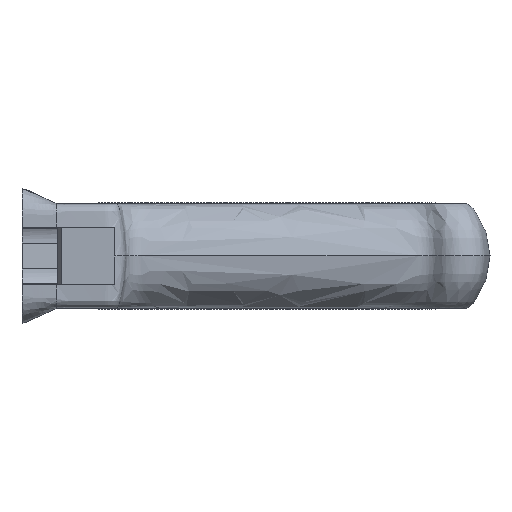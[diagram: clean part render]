
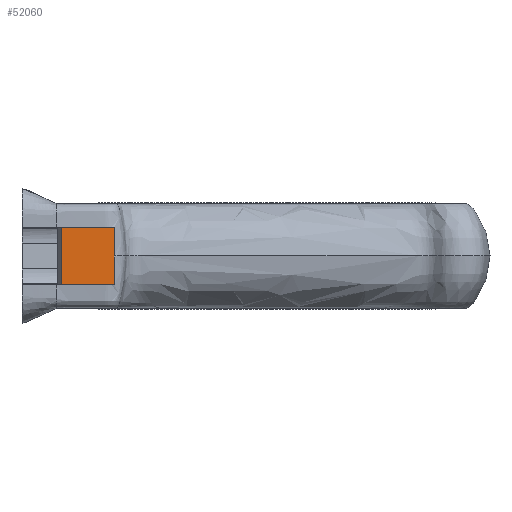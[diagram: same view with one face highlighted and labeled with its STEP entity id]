
A CAD part, left-side view. The second image highlights one B-rep face of the part: STEP entity #52060.
In plain terms, the highlighted planar face has unit normal (-1, 0, 0).
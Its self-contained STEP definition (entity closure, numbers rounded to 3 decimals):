
#742 = LINE ( 'NONE', #743, #13379 ) ;
#743 = CARTESIAN_POINT ( 'NONE',  ( 1.75, -12.5, -6.25 ) ) ;
#744 = DIRECTION ( 'NONE',  ( 0., 1., 0. ) ) ;
#745 = LINE ( 'NONE', #746, #13381 ) ;
#746 = CARTESIAN_POINT ( 'NONE',  ( 1.75, -1.057, -6.25 ) ) ;
#747 = DIRECTION ( 'NONE',  ( 0., 0., 1. ) ) ;
#748 = LINE ( 'NONE', #749, #13384 ) ;
#749 = CARTESIAN_POINT ( 'NONE',  ( 1.75, -12.5, -6.25 ) ) ;
#750 = DIRECTION ( 'NONE',  ( 0., 0., -1. ) ) ;
#751 = LINE ( 'NONE', #752, #13386 ) ;
#752 = CARTESIAN_POINT ( 'NONE',  ( 1.75, -12.5, 6.25 ) ) ;
#753 = DIRECTION ( 'NONE',  ( 0., 1., 0. ) ) ;
#5566 = PLANE ( 'NONE',  #14599 ) ;
#5568 = CARTESIAN_POINT ( 'NONE',  ( 1.75, -12.5, -6.25 ) ) ;
#5570 = DIRECTION ( 'NONE',  ( 1., 0., 0. ) ) ;
#5572 = DIRECTION ( 'NONE',  ( 0., 0., -1. ) ) ;
#13379 = VECTOR ( 'NONE', #744, 1000. ) ;
#13381 = VECTOR ( 'NONE', #747, 1000. ) ;
#13384 = VECTOR ( 'NONE', #750, 1000. ) ;
#13386 = VECTOR ( 'NONE', #753, 1000. ) ;
#14597 = FACE_OUTER_BOUND ( 'NONE', #68502, .T. ) ;
#14599 = AXIS2_PLACEMENT_3D ( 'NONE', #5568, #5570, #5572 ) ;
#48506 = VERTEX_POINT ( 'NONE', #73173 ) ;
#49439 = ORIENTED_EDGE ( 'NONE', *, *, #55894, .T. ) ;
#49500 = ORIENTED_EDGE ( 'NONE', *, *, #55891, .F. ) ;
#49536 = ORIENTED_EDGE ( 'NONE', *, *, #55893, .F. ) ;
#49616 = ORIENTED_EDGE ( 'NONE', *, *, #55892, .F. ) ;
#49675 = VERTEX_POINT ( 'NONE', #73376 ) ;
#49711 = VERTEX_POINT ( 'NONE', #73392 ) ;
#50057 = VERTEX_POINT ( 'NONE', #73529 ) ;
#52060 = ADVANCED_FACE ( 'NONE', ( #14597 ), #5566, .F. ) ;
#55891 = EDGE_CURVE ( 'NONE', #49675, #49711, #742, .T. ) ;
#55892 = EDGE_CURVE ( 'NONE', #49711, #48506, #745, .T. ) ;
#55893 = EDGE_CURVE ( 'NONE', #50057, #49675, #748, .T. ) ;
#55894 = EDGE_CURVE ( 'NONE', #50057, #48506, #751, .T. ) ;
#68502 = EDGE_LOOP ( 'NONE', ( #49616, #49500, #49536, #49439 ) ) ;
#73173 = CARTESIAN_POINT ( 'NONE',  ( 1.75, -1.057, 6.25 ) ) ;
#73376 = CARTESIAN_POINT ( 'NONE',  ( 1.75, -12.5, -6.25 ) ) ;
#73392 = CARTESIAN_POINT ( 'NONE',  ( 1.75, -1.057, -6.25 ) ) ;
#73529 = CARTESIAN_POINT ( 'NONE',  ( 1.75, -12.5, 6.25 ) ) ;
